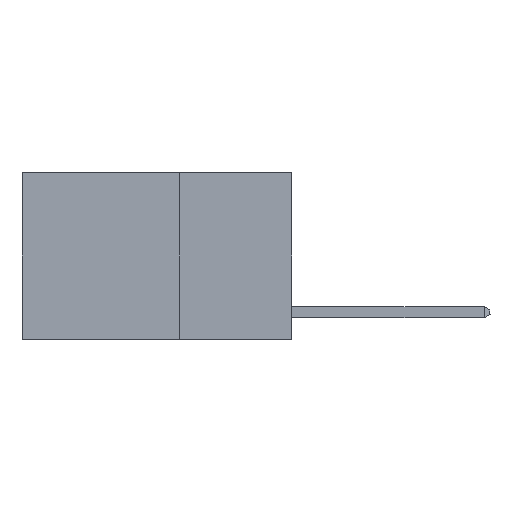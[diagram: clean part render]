
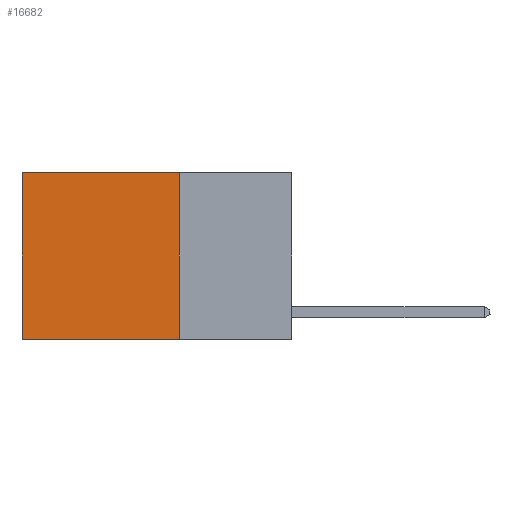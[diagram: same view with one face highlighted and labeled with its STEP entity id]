
A CAD part, left-side view. The second image highlights one B-rep face of the part: STEP entity #16682.
In plain terms, the highlighted planar face has unit normal (-1, 0, 0).
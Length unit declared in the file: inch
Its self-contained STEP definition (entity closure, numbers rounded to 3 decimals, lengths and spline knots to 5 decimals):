
#313 = EDGE_CURVE ( 'NONE', #14629, #15450, #21674, .T. ) ;
#1532 = CARTESIAN_POINT ( 'NONE',  ( 0.2625, 0.6, 0. ) ) ;
#1927 = LINE ( 'NONE', #7882, #25484 ) ;
#3152 = DIRECTION ( 'NONE',  ( 0., 1., 0. ) ) ;
#3364 = ORIENTED_EDGE ( 'NONE', *, *, #313, .F. ) ;
#3693 = VECTOR ( 'NONE', #21734, 39.37008 ) ;
#3854 = DIRECTION ( 'NONE',  ( 1., 0., 0. ) ) ;
#4222 = VERTEX_POINT ( 'NONE', #1532 ) ;
#5668 = DIRECTION ( 'NONE',  ( 0., 1., 0. ) ) ;
#6792 = EDGE_CURVE ( 'NONE', #15450, #13892, #1927, .T. ) ;
#7404 = EDGE_CURVE ( 'NONE', #4222, #13892, #26505, .T. ) ;
#7882 = CARTESIAN_POINT ( 'NONE',  ( 0.2625, 0.25, -0.37 ) ) ;
#8079 = CARTESIAN_POINT ( 'NONE',  ( 0.2625, 0.6, 0. ) ) ;
#9544 = VECTOR ( 'NONE', #28644, 39.37008 ) ;
#9609 = ORIENTED_EDGE ( 'NONE', *, *, #6792, .F. ) ;
#10835 = EDGE_CURVE ( 'NONE', #14629, #4222, #24933, .T. ) ;
#12136 = VECTOR ( 'NONE', #3152, 39.37008 ) ;
#12752 = CARTESIAN_POINT ( 'NONE',  ( 0.2625, 0.25, 0. ) ) ;
#12755 = CARTESIAN_POINT ( 'NONE',  ( 0.2625, 0.25, 0. ) ) ;
#13772 = ORIENTED_EDGE ( 'NONE', *, *, #7404, .T. ) ;
#13892 = VERTEX_POINT ( 'NONE', #14782 ) ;
#14629 = VERTEX_POINT ( 'NONE', #12755 ) ;
#14782 = CARTESIAN_POINT ( 'NONE',  ( 0.2625, 0.6, -0.37 ) ) ;
#15450 = VERTEX_POINT ( 'NONE', #24639 ) ;
#16682 = ADVANCED_FACE ( 'NONE', ( #20415 ), #28851, .F. ) ;
#16849 = ORIENTED_EDGE ( 'NONE', *, *, #10835, .T. ) ;
#17585 = CARTESIAN_POINT ( 'NONE',  ( 0.2625, 0.25, 0. ) ) ;
#19091 = CARTESIAN_POINT ( 'NONE',  ( 0.2625, 0.25, 0. ) ) ;
#19881 = DIRECTION ( 'NONE',  ( 0., 0., -1. ) ) ;
#20415 = FACE_OUTER_BOUND ( 'NONE', #28923, .T. ) ;
#21674 = LINE ( 'NONE', #12752, #9544 ) ;
#21734 = DIRECTION ( 'NONE',  ( 0., 0., -1. ) ) ;
#24639 = CARTESIAN_POINT ( 'NONE',  ( 0.2625, 0.25, -0.37 ) ) ;
#24933 = LINE ( 'NONE', #19091, #12136 ) ;
#25484 = VECTOR ( 'NONE', #5668, 39.37008 ) ;
#25551 = AXIS2_PLACEMENT_3D ( 'NONE', #17585, #3854, #19881 ) ;
#26505 = LINE ( 'NONE', #8079, #3693 ) ;
#28644 = DIRECTION ( 'NONE',  ( 0., 0., -1. ) ) ;
#28851 = PLANE ( 'NONE',  #25551 ) ;
#28923 = EDGE_LOOP ( 'NONE', ( #13772, #9609, #3364, #16849 ) ) ;
